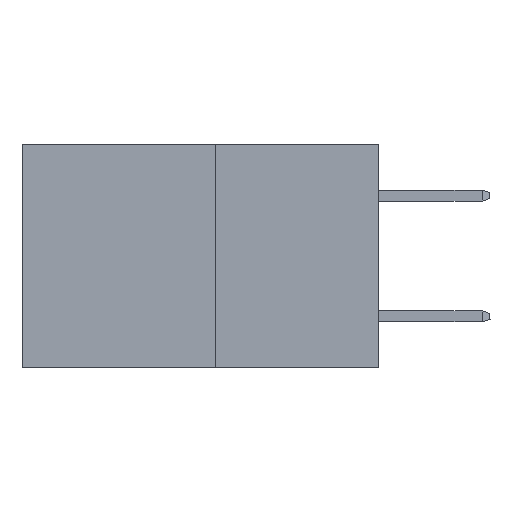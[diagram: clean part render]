
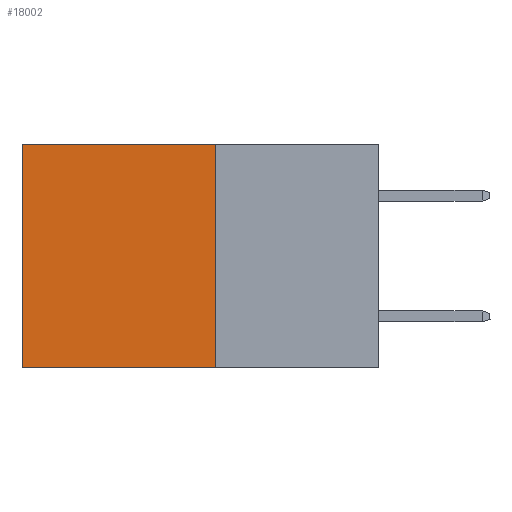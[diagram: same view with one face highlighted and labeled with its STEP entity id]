
A CAD part, left-side view. The second image highlights one B-rep face of the part: STEP entity #18002.
In plain terms, the highlighted planar face has unit normal (-1, 0, 0).
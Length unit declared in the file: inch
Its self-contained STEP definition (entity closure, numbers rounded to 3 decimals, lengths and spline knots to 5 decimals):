
#1745 = VECTOR ( 'NONE', #12937, 39.37008 ) ;
#2065 = VERTEX_POINT ( 'NONE', #20404 ) ;
#3274 = CARTESIAN_POINT ( 'NONE',  ( 0.277, 0.59, 0. ) ) ;
#4861 = ORIENTED_EDGE ( 'NONE', *, *, #12057, .F. ) ;
#8570 = EDGE_CURVE ( 'NONE', #25384, #10156, #28603, .T. ) ;
#8745 = LINE ( 'NONE', #10639, #1745 ) ;
#8810 = DIRECTION ( 'NONE',  ( 0., 1., 0. ) ) ;
#8915 = FACE_OUTER_BOUND ( 'NONE', #16000, .T. ) ;
#9393 = CARTESIAN_POINT ( 'NONE',  ( 0.277, 0.27, -0.37 ) ) ;
#9721 = CARTESIAN_POINT ( 'NONE',  ( 0.277, 0.27, 0. ) ) ;
#10156 = VERTEX_POINT ( 'NONE', #3274 ) ;
#10504 = VECTOR ( 'NONE', #22035, 39.37008 ) ;
#10639 = CARTESIAN_POINT ( 'NONE',  ( 0.277, 0.27, -0.37 ) ) ;
#11728 = DIRECTION ( 'NONE',  ( 1., 0., 0. ) ) ;
#12057 = EDGE_CURVE ( 'NONE', #25384, #2065, #16501, .T. ) ;
#12937 = DIRECTION ( 'NONE',  ( 0., 1., 0. ) ) ;
#13478 = LINE ( 'NONE', #19975, #19444 ) ;
#16000 = EDGE_LOOP ( 'NONE', ( #17062, #27698, #4861, #18813 ) ) ;
#16501 = LINE ( 'NONE', #17465, #10504 ) ;
#17062 = ORIENTED_EDGE ( 'NONE', *, *, #23723, .T. ) ;
#17465 = CARTESIAN_POINT ( 'NONE',  ( 0.277, 0.27, -0.37 ) ) ;
#18002 = ADVANCED_FACE ( 'NONE', ( #8915 ), #22966, .F. ) ;
#18813 = ORIENTED_EDGE ( 'NONE', *, *, #8570, .T. ) ;
#19275 = CARTESIAN_POINT ( 'NONE',  ( 0.277, 0.59, -0.37 ) ) ;
#19444 = VECTOR ( 'NONE', #19876, 39.37008 ) ;
#19876 = DIRECTION ( 'NONE',  ( 0., 0., -1. ) ) ;
#19975 = CARTESIAN_POINT ( 'NONE',  ( 0.277, 0.59, -0.37 ) ) ;
#20404 = CARTESIAN_POINT ( 'NONE',  ( 0.277, 0.27, -0.37 ) ) ;
#20659 = EDGE_CURVE ( 'NONE', #2065, #24814, #8745, .T. ) ;
#22035 = DIRECTION ( 'NONE',  ( 0., 0., -1. ) ) ;
#22581 = VECTOR ( 'NONE', #8810, 39.37008 ) ;
#22966 = PLANE ( 'NONE',  #28409 ) ;
#23723 = EDGE_CURVE ( 'NONE', #10156, #24814, #13478, .T. ) ;
#24814 = VERTEX_POINT ( 'NONE', #19275 ) ;
#25384 = VERTEX_POINT ( 'NONE', #25854 ) ;
#25854 = CARTESIAN_POINT ( 'NONE',  ( 0.277, 0.27, 0. ) ) ;
#27499 = DIRECTION ( 'NONE',  ( 0., 0., -1. ) ) ;
#27698 = ORIENTED_EDGE ( 'NONE', *, *, #20659, .F. ) ;
#28409 = AXIS2_PLACEMENT_3D ( 'NONE', #9393, #11728, #27499 ) ;
#28603 = LINE ( 'NONE', #9721, #22581 ) ;
